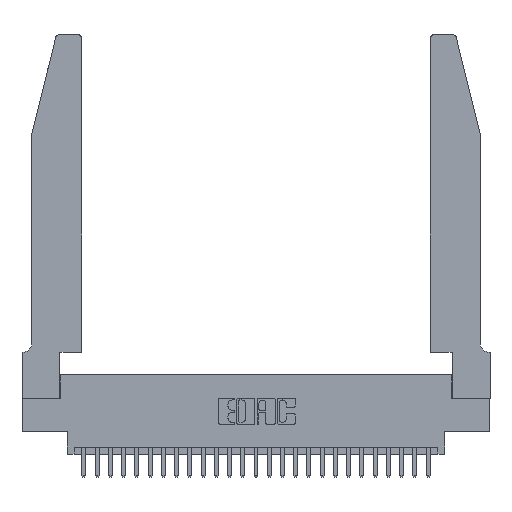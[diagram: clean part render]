
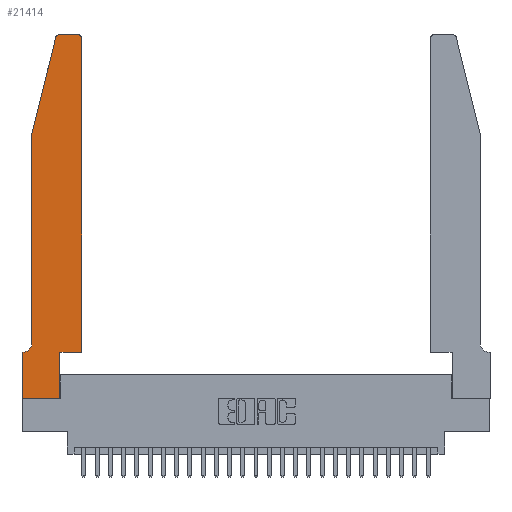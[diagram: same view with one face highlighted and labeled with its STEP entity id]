
A CAD part, top view. The second image highlights one B-rep face of the part: STEP entity #21414.
In plain terms, the highlighted planar face has unit normal (0, 0, 1).
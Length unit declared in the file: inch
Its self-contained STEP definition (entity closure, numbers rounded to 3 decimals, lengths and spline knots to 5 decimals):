
#54 = VERTEX_POINT ( 'NONE', #1698 ) ;
#285 = ORIENTED_EDGE ( 'NONE', *, *, #2793, .T. ) ;
#324 = LINE ( 'NONE', #15543, #4179 ) ;
#705 = CARTESIAN_POINT ( 'NONE',  ( 0., 0.35, 0.37 ) ) ;
#727 = DIRECTION ( 'NONE',  ( 1., 0., 0. ) ) ;
#854 = DIRECTION ( 'NONE',  ( 1., 0., 0. ) ) ;
#1248 = LINE ( 'NONE', #5365, #1949 ) ;
#1685 = CARTESIAN_POINT ( 'NONE',  ( 0.0055, 0.35, 0.37 ) ) ;
#1698 = CARTESIAN_POINT ( 'NONE',  ( 0., 0., 0.37 ) ) ;
#1784 = EDGE_CURVE ( 'NONE', #22313, #2230, #24449, .T. ) ;
#1949 = VECTOR ( 'NONE', #854, 39.37008 ) ;
#2211 = ORIENTED_EDGE ( 'NONE', *, *, #1784, .T. ) ;
#2230 = VERTEX_POINT ( 'NONE', #10665 ) ;
#2235 = EDGE_CURVE ( 'NONE', #7080, #27906, #7854, .T. ) ;
#2265 = EDGE_CURVE ( 'NONE', #12928, #22995, #24419, .T. ) ;
#2567 = DIRECTION ( 'NONE',  ( 0., 0., 1. ) ) ;
#2793 = EDGE_CURVE ( 'NONE', #22995, #22313, #22338, .T. ) ;
#3064 = EDGE_CURVE ( 'NONE', #7930, #27019, #21317, .T. ) ;
#3798 = EDGE_CURVE ( 'NONE', #24921, #7080, #15169, .T. ) ;
#3844 = ORIENTED_EDGE ( 'NONE', *, *, #11239, .T. ) ;
#3961 = CARTESIAN_POINT ( 'NONE',  ( 0.0755, 2., 0.37 ) ) ;
#4179 = VECTOR ( 'NONE', #26348, 39.37008 ) ;
#4183 = CARTESIAN_POINT ( 'NONE',  ( 0.4505, 0.35, 0.37 ) ) ;
#4359 = EDGE_LOOP ( 'NONE', ( #2211, #13839, #10813, #14189, #6452, #5302, #3844, #26406, #17957, #19580, #23141, #285 ) ) ;
#5302 = ORIENTED_EDGE ( 'NONE', *, *, #22391, .T. ) ;
#5365 = CARTESIAN_POINT ( 'NONE',  ( 0.4505, 0.35, 0.37 ) ) ;
#5965 = DIRECTION ( 'NONE',  ( 0., 0., 1. ) ) ;
#6359 = VERTEX_POINT ( 'NONE', #21588 ) ;
#6452 = ORIENTED_EDGE ( 'NONE', *, *, #2235, .T. ) ;
#7080 = VERTEX_POINT ( 'NONE', #19659 ) ;
#7854 = CIRCLE ( 'NONE', #22072, 0.07 ) ;
#7930 = VERTEX_POINT ( 'NONE', #15899 ) ;
#8677 = CARTESIAN_POINT ( 'NONE',  ( 0.0755, 2., 0.37 ) ) ;
#9427 = VECTOR ( 'NONE', #27917, 39.37008 ) ;
#10665 = CARTESIAN_POINT ( 'NONE',  ( 0.284, 2.75, 0.37 ) ) ;
#10813 = ORIENTED_EDGE ( 'NONE', *, *, #24506, .T. ) ;
#11226 = EDGE_CURVE ( 'NONE', #54, #7930, #22953, .T. ) ;
#11239 = EDGE_CURVE ( 'NONE', #25255, #54, #22267, .T. ) ;
#11425 = VECTOR ( 'NONE', #13065, 39.37008 ) ;
#12928 = VERTEX_POINT ( 'NONE', #24386 ) ;
#13065 = DIRECTION ( 'NONE',  ( 1., 0., 0. ) ) ;
#13134 = VECTOR ( 'NONE', #25986, 39.37008 ) ;
#13504 = EDGE_CURVE ( 'NONE', #2230, #6359, #18826, .T. ) ;
#13577 = VECTOR ( 'NONE', #17738, 39.37008 ) ;
#13818 = DIRECTION ( 'NONE',  ( 0., 0., 1. ) ) ;
#13839 = ORIENTED_EDGE ( 'NONE', *, *, #13504, .T. ) ;
#13926 = CARTESIAN_POINT ( 'NONE',  ( 0.4505, 2.72, 0.37 ) ) ;
#14189 = ORIENTED_EDGE ( 'NONE', *, *, #3798, .T. ) ;
#14243 = VECTOR ( 'NONE', #23558, 39.37008 ) ;
#14547 = CARTESIAN_POINT ( 'NONE',  ( 0., 0.35, 0.37 ) ) ;
#14578 = DIRECTION ( 'NONE',  ( 0., 1., 0. ) ) ;
#15060 = CARTESIAN_POINT ( 'NONE',  ( 0., 0., 0.37 ) ) ;
#15169 = LINE ( 'NONE', #25724, #9427 ) ;
#15543 = CARTESIAN_POINT ( 'NONE',  ( 0.0755, 0.35, 0.37 ) ) ;
#15640 = CARTESIAN_POINT ( 'NONE',  ( 0.284, 2.72, 0.37 ) ) ;
#15899 = CARTESIAN_POINT ( 'NONE',  ( 0.2865, 0., 0.37 ) ) ;
#16525 = VECTOR ( 'NONE', #26049, 39.37008 ) ;
#17738 = DIRECTION ( 'NONE',  ( -1., 0., 0. ) ) ;
#17846 = DIRECTION ( 'NONE',  ( 1., 0., 0. ) ) ;
#17957 = ORIENTED_EDGE ( 'NONE', *, *, #3064, .T. ) ;
#17970 = CARTESIAN_POINT ( 'NONE',  ( 0.2865, 0.35, 0.37 ) ) ;
#18826 = CIRCLE ( 'NONE', #27895, 0.03 ) ;
#18937 = LINE ( 'NONE', #8677, #13134 ) ;
#18939 = PLANE ( 'NONE',  #21399 ) ;
#19580 = ORIENTED_EDGE ( 'NONE', *, *, #24228, .T. ) ;
#19659 = CARTESIAN_POINT ( 'NONE',  ( 0.0755, 0.42, 0.37 ) ) ;
#21088 = DIRECTION ( 'NONE',  ( 1., 0., 0. ) ) ;
#21317 = LINE ( 'NONE', #25380, #26402 ) ;
#21399 = AXIS2_PLACEMENT_3D ( 'NONE', #14547, #5965, #21088 ) ;
#21414 = ADVANCED_FACE ( 'NONE', ( #21838 ), #18939, .T. ) ;
#21588 = CARTESIAN_POINT ( 'NONE',  ( 0.25487, 2.72718, 0.37 ) ) ;
#21838 = FACE_OUTER_BOUND ( 'NONE', #4359, .T. ) ;
#22072 = AXIS2_PLACEMENT_3D ( 'NONE', #28180, #28078, #27484 ) ;
#22267 = LINE ( 'NONE', #15060, #16525 ) ;
#22313 = VERTEX_POINT ( 'NONE', #23991 ) ;
#22338 = CIRCLE ( 'NONE', #24441, 0.03 ) ;
#22391 = EDGE_CURVE ( 'NONE', #27906, #25255, #324, .T. ) ;
#22953 = LINE ( 'NONE', #26709, #11425 ) ;
#22969 = CARTESIAN_POINT ( 'NONE',  ( 0.2605, 2.75, 0.37 ) ) ;
#22995 = VERTEX_POINT ( 'NONE', #13926 ) ;
#23141 = ORIENTED_EDGE ( 'NONE', *, *, #2265, .T. ) ;
#23558 = DIRECTION ( 'NONE',  ( 0., 1., 0. ) ) ;
#23991 = CARTESIAN_POINT ( 'NONE',  ( 0.4205, 2.75, 0.37 ) ) ;
#24228 = EDGE_CURVE ( 'NONE', #27019, #12928, #1248, .T. ) ;
#24386 = CARTESIAN_POINT ( 'NONE',  ( 0.4505, 0.35, 0.37 ) ) ;
#24419 = LINE ( 'NONE', #4183, #14243 ) ;
#24441 = AXIS2_PLACEMENT_3D ( 'NONE', #26817, #13818, #727 ) ;
#24449 = LINE ( 'NONE', #22969, #13577 ) ;
#24506 = EDGE_CURVE ( 'NONE', #6359, #24921, #18937, .T. ) ;
#24921 = VERTEX_POINT ( 'NONE', #3961 ) ;
#25255 = VERTEX_POINT ( 'NONE', #705 ) ;
#25380 = CARTESIAN_POINT ( 'NONE',  ( 0.2865, 0.35, 0.37 ) ) ;
#25724 = CARTESIAN_POINT ( 'NONE',  ( 0.0755, 2., 0.37 ) ) ;
#25986 = DIRECTION ( 'NONE',  ( -0.239, -0.971, 0. ) ) ;
#26049 = DIRECTION ( 'NONE',  ( 0., -1., 0. ) ) ;
#26348 = DIRECTION ( 'NONE',  ( -1., 0., 0. ) ) ;
#26402 = VECTOR ( 'NONE', #14578, 39.37008 ) ;
#26406 = ORIENTED_EDGE ( 'NONE', *, *, #11226, .T. ) ;
#26709 = CARTESIAN_POINT ( 'NONE',  ( 0., 0., 0.37 ) ) ;
#26817 = CARTESIAN_POINT ( 'NONE',  ( 0.4205, 2.72, 0.37 ) ) ;
#27019 = VERTEX_POINT ( 'NONE', #17970 ) ;
#27484 = DIRECTION ( 'NONE',  ( -1., 0., 0. ) ) ;
#27895 = AXIS2_PLACEMENT_3D ( 'NONE', #15640, #2567, #17846 ) ;
#27906 = VERTEX_POINT ( 'NONE', #1685 ) ;
#27917 = DIRECTION ( 'NONE',  ( 0., -1., 0. ) ) ;
#28078 = DIRECTION ( 'NONE',  ( 0., 0., -1. ) ) ;
#28180 = CARTESIAN_POINT ( 'NONE',  ( 0.0055, 0.42, 0.37 ) ) ;
